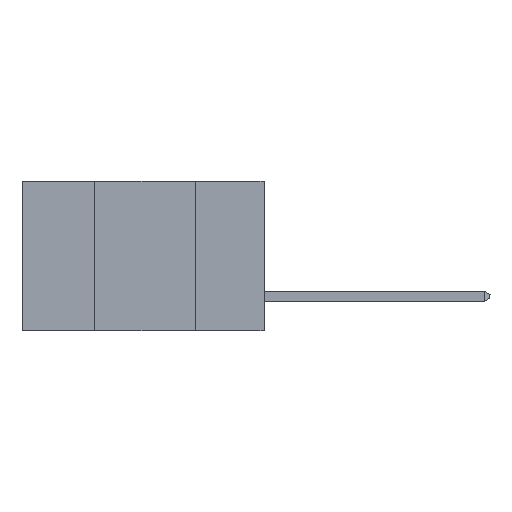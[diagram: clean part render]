
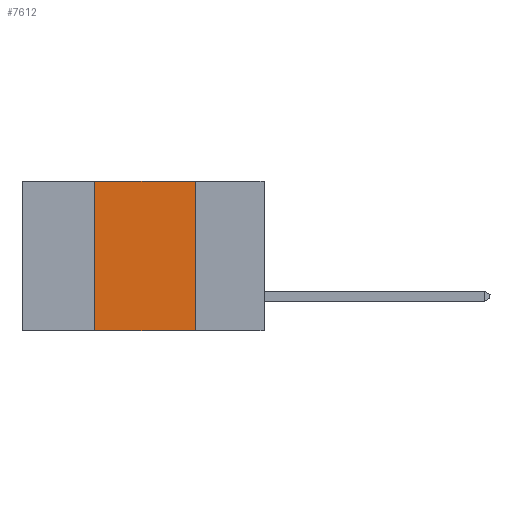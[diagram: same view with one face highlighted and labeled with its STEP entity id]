
A CAD part, left-side view. The second image highlights one B-rep face of the part: STEP entity #7612.
In plain terms, the highlighted planar face has unit normal (-1, 0, 0).
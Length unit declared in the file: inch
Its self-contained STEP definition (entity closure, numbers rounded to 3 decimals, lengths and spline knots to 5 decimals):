
#113 = ORIENTED_EDGE ( 'NONE', *, *, #2636, .T. ) ;
#819 = CARTESIAN_POINT ( 'NONE',  ( 0., 0.6, -0.37 ) ) ;
#875 = CARTESIAN_POINT ( 'NONE',  ( 0., 0.6, 0. ) ) ;
#1150 = ORIENTED_EDGE ( 'NONE', *, *, #5543, .F. ) ;
#1285 = EDGE_LOOP ( 'NONE', ( #1150, #14107, #9031, #113 ) ) ;
#1464 = DIRECTION ( 'NONE',  ( 1., 0., 0. ) ) ;
#1491 = VERTEX_POINT ( 'NONE', #8385 ) ;
#1747 = LINE ( 'NONE', #1913, #7166 ) ;
#1820 = EDGE_CURVE ( 'NONE', #14168, #2406, #14827, .T. ) ;
#1913 = CARTESIAN_POINT ( 'NONE',  ( 0., 0.17, -0.37 ) ) ;
#2406 = VERTEX_POINT ( 'NONE', #5395 ) ;
#2463 = FACE_OUTER_BOUND ( 'NONE', #1285, .T. ) ;
#2636 = EDGE_CURVE ( 'NONE', #1491, #2922, #4714, .T. ) ;
#2657 = VECTOR ( 'NONE', #13740, 39.37008 ) ;
#2922 = VERTEX_POINT ( 'NONE', #8131 ) ;
#4714 = LINE ( 'NONE', #819, #5831 ) ;
#5395 = CARTESIAN_POINT ( 'NONE',  ( 0., 0.17, 0. ) ) ;
#5543 = EDGE_CURVE ( 'NONE', #2406, #2922, #1747, .T. ) ;
#5823 = DIRECTION ( 'NONE',  ( 0., 0., -1. ) ) ;
#5831 = VECTOR ( 'NONE', #6047, 39.37008 ) ;
#6019 = LINE ( 'NONE', #15246, #2657 ) ;
#6047 = DIRECTION ( 'NONE',  ( 0., -1., 0. ) ) ;
#6191 = EDGE_CURVE ( 'NONE', #1491, #14168, #6019, .T. ) ;
#6459 = DIRECTION ( 'NONE',  ( 0., 0., -1. ) ) ;
#7166 = VECTOR ( 'NONE', #5823, 39.37008 ) ;
#7612 = ADVANCED_FACE ( 'NONE', ( #2463 ), #15519, .F. ) ;
#8131 = CARTESIAN_POINT ( 'NONE',  ( 0., 0.17, -0.37 ) ) ;
#8385 = CARTESIAN_POINT ( 'NONE',  ( 0., 0.42, -0.37 ) ) ;
#9031 = ORIENTED_EDGE ( 'NONE', *, *, #6191, .F. ) ;
#10364 = CARTESIAN_POINT ( 'NONE',  ( 0., 0.42, 0. ) ) ;
#12262 = DIRECTION ( 'NONE',  ( 0., -1., 0. ) ) ;
#12499 = AXIS2_PLACEMENT_3D ( 'NONE', #12856, #1464, #6459 ) ;
#12856 = CARTESIAN_POINT ( 'NONE',  ( 0., 0.6, 0. ) ) ;
#13740 = DIRECTION ( 'NONE',  ( 0., 0., 1. ) ) ;
#14107 = ORIENTED_EDGE ( 'NONE', *, *, #1820, .F. ) ;
#14168 = VERTEX_POINT ( 'NONE', #10364 ) ;
#14827 = LINE ( 'NONE', #875, #15900 ) ;
#15246 = CARTESIAN_POINT ( 'NONE',  ( 0., 0.42, -0.37 ) ) ;
#15519 = PLANE ( 'NONE',  #12499 ) ;
#15900 = VECTOR ( 'NONE', #12262, 39.37008 ) ;
